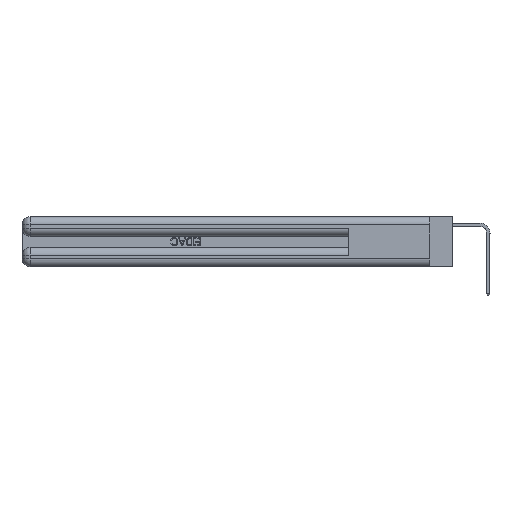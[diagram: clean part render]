
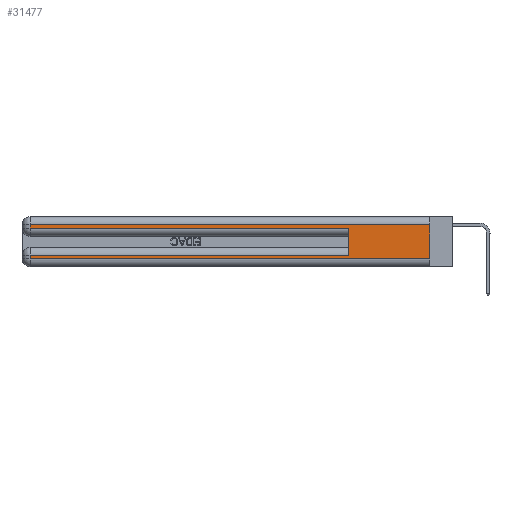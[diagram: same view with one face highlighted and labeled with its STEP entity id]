
A CAD part, left-side view. The second image highlights one B-rep face of the part: STEP entity #31477.
In plain terms, the highlighted planar face has unit normal (-1, 0, 0).
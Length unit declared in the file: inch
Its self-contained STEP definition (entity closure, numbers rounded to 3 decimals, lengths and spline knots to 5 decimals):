
#464 = CARTESIAN_POINT ( 'NONE',  ( 0., 0., 0.37 ) ) ;
#793 = CARTESIAN_POINT ( 'NONE',  ( 0., 0., 0.31 ) ) ;
#816 = CARTESIAN_POINT ( 'NONE',  ( 0., 2.94, 0.37 ) ) ;
#2452 = CARTESIAN_POINT ( 'NONE',  ( 0., 0.6, 0.145 ) ) ;
#2532 = DIRECTION ( 'NONE',  ( 0., 1., 0. ) ) ;
#2815 = CARTESIAN_POINT ( 'NONE',  ( 0., 0., 0.06 ) ) ;
#3084 = VECTOR ( 'NONE', #20002, 39.37008 ) ;
#3272 = DIRECTION ( 'NONE',  ( 1., 0., 0. ) ) ;
#4247 = ORIENTED_EDGE ( 'NONE', *, *, #21349, .T. ) ;
#6294 = ORIENTED_EDGE ( 'NONE', *, *, #25430, .T. ) ;
#7744 = LINE ( 'NONE', #29777, #14196 ) ;
#8050 = DIRECTION ( 'NONE',  ( 0., -1., 0. ) ) ;
#8188 = CARTESIAN_POINT ( 'NONE',  ( 0., 2.94, 0.085 ) ) ;
#8801 = AXIS2_PLACEMENT_3D ( 'NONE', #464, #3272, #22439 ) ;
#8974 = VERTEX_POINT ( 'NONE', #23854 ) ;
#9388 = EDGE_CURVE ( 'NONE', #26615, #12389, #25698, .T. ) ;
#9678 = VERTEX_POINT ( 'NONE', #18741 ) ;
#10181 = EDGE_LOOP ( 'NONE', ( #16698, #21697, #4247, #22083, #11885, #6294, #33331, #34834 ) ) ;
#10210 = EDGE_CURVE ( 'NONE', #8974, #22655, #7744, .T. ) ;
#11199 = VECTOR ( 'NONE', #31028, 39.37008 ) ;
#11430 = EDGE_CURVE ( 'NONE', #19998, #22655, #14528, .T. ) ;
#11506 = EDGE_CURVE ( 'NONE', #12389, #9678, #33640, .T. ) ;
#11813 = CARTESIAN_POINT ( 'NONE',  ( 0., 0., 0.37 ) ) ;
#11885 = ORIENTED_EDGE ( 'NONE', *, *, #11430, .F. ) ;
#11998 = CARTESIAN_POINT ( 'NONE',  ( 0., 2.94, 0.37 ) ) ;
#12322 = FACE_OUTER_BOUND ( 'NONE', #10181, .T. ) ;
#12389 = VERTEX_POINT ( 'NONE', #28464 ) ;
#13677 = VECTOR ( 'NONE', #18835, 39.37008 ) ;
#13897 = CARTESIAN_POINT ( 'NONE',  ( 0., 0.6, 0.085 ) ) ;
#14196 = VECTOR ( 'NONE', #8050, 39.37008 ) ;
#14528 = LINE ( 'NONE', #2452, #13677 ) ;
#14547 = DIRECTION ( 'NONE',  ( 0., 0., -1. ) ) ;
#14657 = EDGE_CURVE ( 'NONE', #29411, #16061, #22072, .T. ) ;
#15103 = DIRECTION ( 'NONE',  ( 0., 1., 0. ) ) ;
#15852 = LINE ( 'NONE', #16174, #22307 ) ;
#16061 = VERTEX_POINT ( 'NONE', #27635 ) ;
#16174 = CARTESIAN_POINT ( 'NONE',  ( 0., 0., 0.085 ) ) ;
#16698 = ORIENTED_EDGE ( 'NONE', *, *, #18915, .F. ) ;
#16920 = VECTOR ( 'NONE', #14547, 39.37008 ) ;
#18741 = CARTESIAN_POINT ( 'NONE',  ( 0., 0., 0.06 ) ) ;
#18835 = DIRECTION ( 'NONE',  ( 0., 0., 1. ) ) ;
#18915 = EDGE_CURVE ( 'NONE', #29411, #9678, #19471, .T. ) ;
#19471 = LINE ( 'NONE', #11813, #16920 ) ;
#19998 = VERTEX_POINT ( 'NONE', #13897 ) ;
#20002 = DIRECTION ( 'NONE',  ( 0., 0., -1. ) ) ;
#21349 = EDGE_CURVE ( 'NONE', #16061, #8974, #31237, .T. ) ;
#21697 = ORIENTED_EDGE ( 'NONE', *, *, #14657, .T. ) ;
#22072 = LINE ( 'NONE', #31375, #30135 ) ;
#22083 = ORIENTED_EDGE ( 'NONE', *, *, #10210, .T. ) ;
#22307 = VECTOR ( 'NONE', #2532, 39.37008 ) ;
#22439 = DIRECTION ( 'NONE',  ( 0., 0., -1. ) ) ;
#22655 = VERTEX_POINT ( 'NONE', #33120 ) ;
#23854 = CARTESIAN_POINT ( 'NONE',  ( 0., 2.94, 0.285 ) ) ;
#24711 = DIRECTION ( 'NONE',  ( 0., -1., 0. ) ) ;
#25430 = EDGE_CURVE ( 'NONE', #19998, #26615, #15852, .T. ) ;
#25605 = VECTOR ( 'NONE', #24711, 39.37008 ) ;
#25698 = LINE ( 'NONE', #11998, #11199 ) ;
#26615 = VERTEX_POINT ( 'NONE', #8188 ) ;
#27635 = CARTESIAN_POINT ( 'NONE',  ( 0., 2.94, 0.31 ) ) ;
#28464 = CARTESIAN_POINT ( 'NONE',  ( 0., 2.94, 0.06 ) ) ;
#29411 = VERTEX_POINT ( 'NONE', #793 ) ;
#29777 = CARTESIAN_POINT ( 'NONE',  ( 0., 0., 0.285 ) ) ;
#30135 = VECTOR ( 'NONE', #15103, 39.37008 ) ;
#31028 = DIRECTION ( 'NONE',  ( 0., 0., -1. ) ) ;
#31237 = LINE ( 'NONE', #816, #3084 ) ;
#31375 = CARTESIAN_POINT ( 'NONE',  ( 0., 0., 0.31 ) ) ;
#31477 = ADVANCED_FACE ( 'NONE', ( #12322 ), #33170, .F. ) ;
#33120 = CARTESIAN_POINT ( 'NONE',  ( 0., 0.6, 0.285 ) ) ;
#33170 = PLANE ( 'NONE',  #8801 ) ;
#33331 = ORIENTED_EDGE ( 'NONE', *, *, #9388, .T. ) ;
#33640 = LINE ( 'NONE', #2815, #25605 ) ;
#34834 = ORIENTED_EDGE ( 'NONE', *, *, #11506, .T. ) ;
